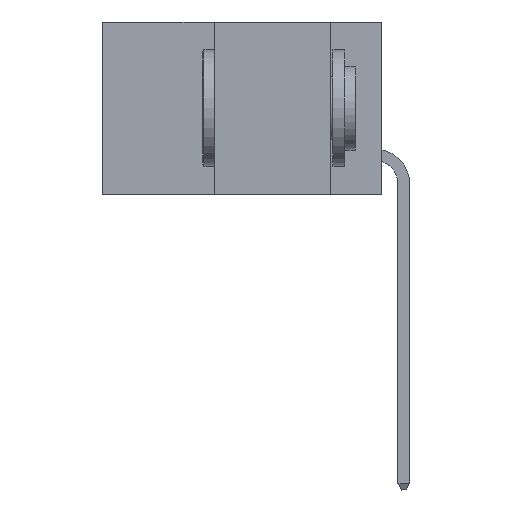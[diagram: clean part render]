
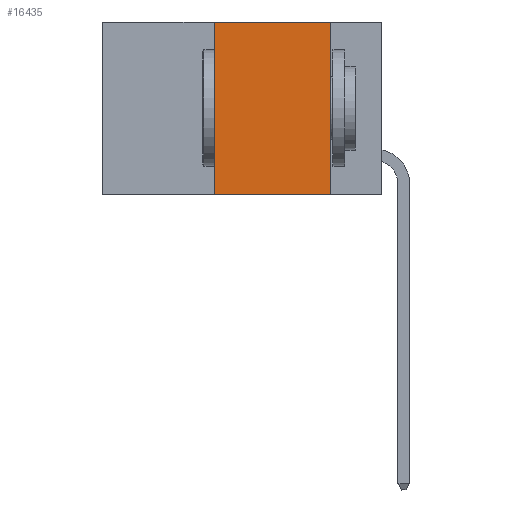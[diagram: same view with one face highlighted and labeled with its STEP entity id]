
A CAD part, left-side view. The second image highlights one B-rep face of the part: STEP entity #16435.
In plain terms, the highlighted planar face has unit normal (-1, 0, 0).
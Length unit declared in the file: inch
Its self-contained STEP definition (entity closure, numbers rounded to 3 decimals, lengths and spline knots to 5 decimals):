
#727 = CARTESIAN_POINT ( 'NONE',  ( 0., 0.36, 0. ) ) ;
#2684 = LINE ( 'NONE', #3976, #16286 ) ;
#3309 = DIRECTION ( 'NONE',  ( 1., 0., 0. ) ) ;
#3881 = LINE ( 'NONE', #16911, #12750 ) ;
#3976 = CARTESIAN_POINT ( 'NONE',  ( 0., 0.6, 0. ) ) ;
#4796 = ORIENTED_EDGE ( 'NONE', *, *, #6465, .T. ) ;
#5156 = CARTESIAN_POINT ( 'NONE',  ( 0., 0.11, 0. ) ) ;
#5429 = EDGE_CURVE ( 'NONE', #16647, #10301, #16307, .T. ) ;
#6465 = EDGE_CURVE ( 'NONE', #9695, #10301, #3881, .T. ) ;
#6515 = CARTESIAN_POINT ( 'NONE',  ( 0., 0.36, -0.37 ) ) ;
#6588 = EDGE_CURVE ( 'NONE', #9695, #9433, #9663, .T. ) ;
#7949 = CARTESIAN_POINT ( 'NONE',  ( 0., 0.36, 0. ) ) ;
#8267 = PLANE ( 'NONE',  #8892 ) ;
#8443 = EDGE_LOOP ( 'NONE', ( #15485, #12271, #14788, #4796 ) ) ;
#8892 = AXIS2_PLACEMENT_3D ( 'NONE', #15133, #3309, #12543 ) ;
#9433 = VERTEX_POINT ( 'NONE', #727 ) ;
#9663 = LINE ( 'NONE', #7949, #11322 ) ;
#9695 = VERTEX_POINT ( 'NONE', #6515 ) ;
#10301 = VERTEX_POINT ( 'NONE', #12740 ) ;
#10411 = CARTESIAN_POINT ( 'NONE',  ( 0., 0.11, 0. ) ) ;
#10957 = VECTOR ( 'NONE', #11787, 39.37008 ) ;
#11322 = VECTOR ( 'NONE', #13109, 39.37008 ) ;
#11640 = EDGE_CURVE ( 'NONE', #9433, #16647, #2684, .T. ) ;
#11787 = DIRECTION ( 'NONE',  ( 0., 0., -1. ) ) ;
#12271 = ORIENTED_EDGE ( 'NONE', *, *, #11640, .F. ) ;
#12543 = DIRECTION ( 'NONE',  ( 0., 0., -1. ) ) ;
#12740 = CARTESIAN_POINT ( 'NONE',  ( 0., 0.11, -0.37 ) ) ;
#12750 = VECTOR ( 'NONE', #15592, 39.37008 ) ;
#13109 = DIRECTION ( 'NONE',  ( 0., 0., 1. ) ) ;
#13201 = DIRECTION ( 'NONE',  ( 0., -1., 0. ) ) ;
#13693 = FACE_OUTER_BOUND ( 'NONE', #8443, .T. ) ;
#14788 = ORIENTED_EDGE ( 'NONE', *, *, #6588, .F. ) ;
#15133 = CARTESIAN_POINT ( 'NONE',  ( 0., 0.6, 0. ) ) ;
#15485 = ORIENTED_EDGE ( 'NONE', *, *, #5429, .F. ) ;
#15592 = DIRECTION ( 'NONE',  ( 0., -1., 0. ) ) ;
#16286 = VECTOR ( 'NONE', #13201, 39.37008 ) ;
#16307 = LINE ( 'NONE', #10411, #10957 ) ;
#16435 = ADVANCED_FACE ( 'NONE', ( #13693 ), #8267, .F. ) ;
#16647 = VERTEX_POINT ( 'NONE', #5156 ) ;
#16911 = CARTESIAN_POINT ( 'NONE',  ( 0., 0.6, -0.37 ) ) ;
